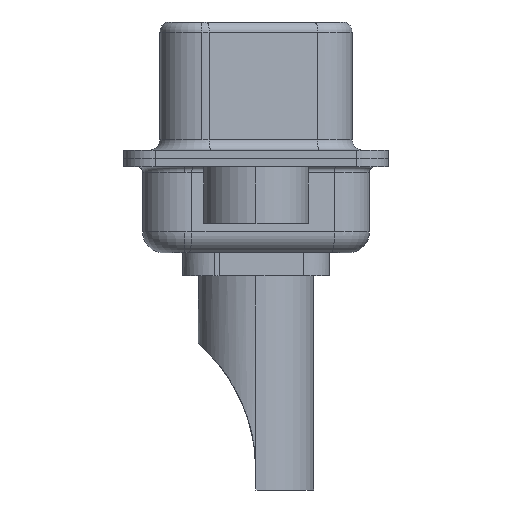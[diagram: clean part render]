
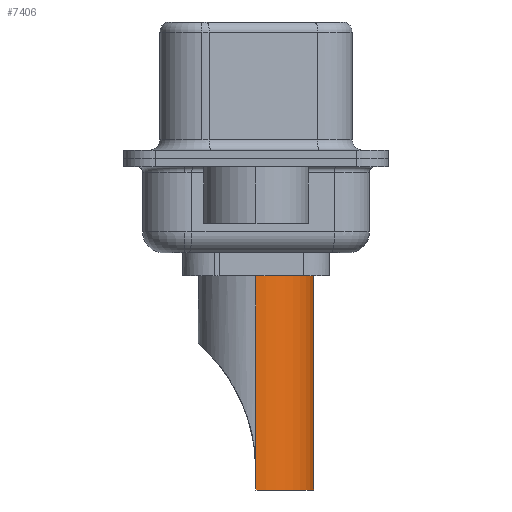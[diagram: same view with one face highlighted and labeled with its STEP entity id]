
A CAD part, left-side view. The second image highlights one B-rep face of the part: STEP entity #7406.
In plain terms, the highlighted cylindrical face has radius 2.75 mm (diameter 5.5 mm), a partial arc.
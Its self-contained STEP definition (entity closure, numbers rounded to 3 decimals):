
#665 = VERTEX_POINT ( 'NONE', #6259 ) ;
#666 = DIRECTION ( 'NONE',  ( 0., 0., 1. ) ) ;
#842 = DIRECTION ( 'NONE',  ( 0., 0., 1. ) ) ;
#1262 = CARTESIAN_POINT ( 'NONE',  ( -2.75, 0., 4.234 ) ) ;
#1290 = VERTEX_POINT ( 'NONE', #15879 ) ;
#1462 = CARTESIAN_POINT ( 'NONE',  ( 2.75, 0., 4.234 ) ) ;
#2956 = DIRECTION ( 'NONE',  ( 0., 0., 1. ) ) ;
#3127 = AXIS2_PLACEMENT_3D ( 'NONE', #6558, #666, #16531 ) ;
#3354 = CYLINDRICAL_SURFACE ( 'NONE', #3127, 2.75 ) ;
#3536 = CARTESIAN_POINT ( 'NONE',  ( -2.75, 0., -8.7 ) ) ;
#3652 = DIRECTION ( 'NONE',  ( 0., 0., 1. ) ) ;
#3726 = DIRECTION ( 'NONE',  ( 0., 0., -1. ) ) ;
#3785 = VECTOR ( 'NONE', #10154, 1000. ) ;
#3823 = FACE_OUTER_BOUND ( 'NONE', #17817, .T. ) ;
#4013 = CIRCLE ( 'NONE', #16470, 2.75 ) ;
#4239 = LINE ( 'NONE', #1262, #3785 ) ;
#4615 = AXIS2_PLACEMENT_3D ( 'NONE', #9641, #842, #11098 ) ;
#4747 = CARTESIAN_POINT ( 'NONE',  ( 2.75, 0., -8.7 ) ) ;
#5126 = CARTESIAN_POINT ( 'NONE',  ( 2.75, 0., -8.7 ) ) ;
#6202 = VERTEX_POINT ( 'NONE', #4747 ) ;
#6259 = CARTESIAN_POINT ( 'NONE',  ( -2.75, 0., 1.5 ) ) ;
#6558 = CARTESIAN_POINT ( 'NONE',  ( 0., 0., 4.234 ) ) ;
#6789 = ORIENTED_EDGE ( 'NONE', *, *, #8463, .T. ) ;
#7026 = CARTESIAN_POINT ( 'NONE',  ( 2.75, 0., -7.764 ) ) ;
#7338 = ORIENTED_EDGE ( 'NONE', *, *, #8349, .F. ) ;
#7406 = ADVANCED_FACE ( 'NONE', ( #3823 ), #3354, .T. ) ;
#7447 = LINE ( 'NONE', #5126, #18169 ) ;
#7659 = VECTOR ( 'NONE', #2956, 1000. ) ;
#7867 = CARTESIAN_POINT ( 'NONE',  ( -2.75, 0., -7.764 ) ) ;
#8337 = VECTOR ( 'NONE', #17756, 1000. ) ;
#8349 = EDGE_CURVE ( 'NONE', #16269, #665, #4239, .T. ) ;
#8379 = EDGE_CURVE ( 'NONE', #15120, #11257, #18376, .T. ) ;
#8462 = ORIENTED_EDGE ( 'NONE', *, *, #8484, .T. ) ;
#8463 = EDGE_CURVE ( 'NONE', #16269, #1290, #9256, .T. ) ;
#8484 = EDGE_CURVE ( 'NONE', #1290, #6202, #4013, .T. ) ;
#8508 = EDGE_CURVE ( 'NONE', #15120, #6202, #7447, .T. ) ;
#8549 = EDGE_CURVE ( 'NONE', #665, #11257, #10350, .T. ) ;
#9256 = LINE ( 'NONE', #3536, #8337 ) ;
#9641 = CARTESIAN_POINT ( 'NONE',  ( 0., 0., 1.5 ) ) ;
#10154 = DIRECTION ( 'NONE',  ( 0., 0., 1. ) ) ;
#10350 = CIRCLE ( 'NONE', #4615, 2.75 ) ;
#11098 = DIRECTION ( 'NONE',  ( 1., 0., 0. ) ) ;
#11257 = VERTEX_POINT ( 'NONE', #11333 ) ;
#11333 = CARTESIAN_POINT ( 'NONE',  ( 2.75, 0., 1.5 ) ) ;
#12378 = CARTESIAN_POINT ( 'NONE',  ( 0., 0., -8.7 ) ) ;
#13807 = DIRECTION ( 'NONE',  ( 1., 0., 0. ) ) ;
#13947 = ORIENTED_EDGE ( 'NONE', *, *, #8549, .F. ) ;
#14371 = ORIENTED_EDGE ( 'NONE', *, *, #8508, .F. ) ;
#15120 = VERTEX_POINT ( 'NONE', #7026 ) ;
#15879 = CARTESIAN_POINT ( 'NONE',  ( -2.75, 0., -8.7 ) ) ;
#16094 = ORIENTED_EDGE ( 'NONE', *, *, #8379, .T. ) ;
#16269 = VERTEX_POINT ( 'NONE', #7867 ) ;
#16470 = AXIS2_PLACEMENT_3D ( 'NONE', #12378, #3652, #13807 ) ;
#16531 = DIRECTION ( 'NONE',  ( 1., 0., 0. ) ) ;
#17756 = DIRECTION ( 'NONE',  ( 0., 0., -1. ) ) ;
#17817 = EDGE_LOOP ( 'NONE', ( #7338, #6789, #8462, #14371, #16094, #13947 ) ) ;
#18169 = VECTOR ( 'NONE', #3726, 1000. ) ;
#18376 = LINE ( 'NONE', #1462, #7659 ) ;
